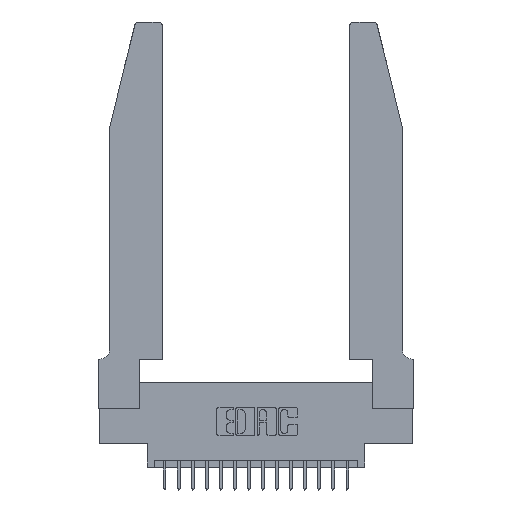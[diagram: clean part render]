
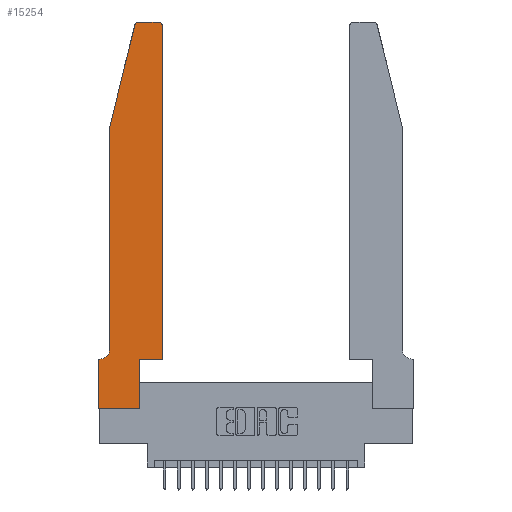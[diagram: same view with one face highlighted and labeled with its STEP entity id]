
A CAD part, top view. The second image highlights one B-rep face of the part: STEP entity #15254.
In plain terms, the highlighted planar face has unit normal (0, 0, 1).
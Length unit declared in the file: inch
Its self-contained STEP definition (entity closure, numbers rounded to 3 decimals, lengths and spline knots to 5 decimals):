
#12 = ORIENTED_EDGE ( 'NONE', *, *, #8720, .T. ) ;
#20 = CARTESIAN_POINT ( 'NONE',  ( 0.4505, 0.35, 0.37 ) ) ;
#29 = CARTESIAN_POINT ( 'NONE',  ( 0.0055, 0.35, 0.37 ) ) ;
#55 = CARTESIAN_POINT ( 'NONE',  ( 0., 0., 0.37 ) ) ;
#153 = LINE ( 'NONE', #2001, #19459 ) ;
#186 = VERTEX_POINT ( 'NONE', #4231 ) ;
#279 = ORIENTED_EDGE ( 'NONE', *, *, #2983, .T. ) ;
#730 = CARTESIAN_POINT ( 'NONE',  ( 0.2865, 0., 0.37 ) ) ;
#1021 = ORIENTED_EDGE ( 'NONE', *, *, #10683, .T. ) ;
#1034 = VERTEX_POINT ( 'NONE', #730 ) ;
#1045 = LINE ( 'NONE', #9131, #12900 ) ;
#1216 = VERTEX_POINT ( 'NONE', #13313 ) ;
#1297 = DIRECTION ( 'NONE',  ( 0., 1., 0. ) ) ;
#1299 = VECTOR ( 'NONE', #12445, 39.37008 ) ;
#1786 = ORIENTED_EDGE ( 'NONE', *, *, #2866, .T. ) ;
#1904 = ORIENTED_EDGE ( 'NONE', *, *, #4023, .T. ) ;
#2001 = CARTESIAN_POINT ( 'NONE',  ( 0., 0., 0.37 ) ) ;
#2242 = ORIENTED_EDGE ( 'NONE', *, *, #8294, .T. ) ;
#2747 = DIRECTION ( 'NONE',  ( -1., 0., 0. ) ) ;
#2837 = DIRECTION ( 'NONE',  ( 0., 0., 1. ) ) ;
#2853 = LINE ( 'NONE', #5395, #6052 ) ;
#2866 = EDGE_CURVE ( 'NONE', #18072, #1216, #2853, .T. ) ;
#2983 = EDGE_CURVE ( 'NONE', #17283, #18072, #4599, .T. ) ;
#3052 = VECTOR ( 'NONE', #2747, 39.37008 ) ;
#3189 = VECTOR ( 'NONE', #18941, 39.37008 ) ;
#3270 = VECTOR ( 'NONE', #19265, 39.37008 ) ;
#3274 = VERTEX_POINT ( 'NONE', #20 ) ;
#3355 = PLANE ( 'NONE',  #6150 ) ;
#3549 = LINE ( 'NONE', #4206, #3052 ) ;
#3795 = DIRECTION ( 'NONE',  ( 1., 0., 0. ) ) ;
#3819 = DIRECTION ( 'NONE',  ( 0., 0., 1. ) ) ;
#3846 = CARTESIAN_POINT ( 'NONE',  ( 0.284, 2.72, 0.37 ) ) ;
#4023 = EDGE_CURVE ( 'NONE', #4287, #186, #3549, .T. ) ;
#4206 = CARTESIAN_POINT ( 'NONE',  ( 0.0755, 0.35, 0.37 ) ) ;
#4231 = CARTESIAN_POINT ( 'NONE',  ( 0., 0.35, 0.37 ) ) ;
#4287 = VERTEX_POINT ( 'NONE', #29 ) ;
#4508 = VERTEX_POINT ( 'NONE', #18841 ) ;
#4599 = CIRCLE ( 'NONE', #12120, 0.03 ) ;
#4802 = CIRCLE ( 'NONE', #5574, 0.07 ) ;
#4921 = FACE_OUTER_BOUND ( 'NONE', #16742, .T. ) ;
#4939 = EDGE_CURVE ( 'NONE', #14732, #1034, #153, .T. ) ;
#4951 = DIRECTION ( 'NONE',  ( 0., 0., 1. ) ) ;
#5345 = DIRECTION ( 'NONE',  ( -0.239, -0.971, 0. ) ) ;
#5395 = CARTESIAN_POINT ( 'NONE',  ( 0.0755, 2., 0.37 ) ) ;
#5574 = AXIS2_PLACEMENT_3D ( 'NONE', #5576, #16064, #7082 ) ;
#5576 = CARTESIAN_POINT ( 'NONE',  ( 0.0055, 0.42, 0.37 ) ) ;
#5972 = AXIS2_PLACEMENT_3D ( 'NONE', #12069, #2837, #13557 ) ;
#6052 = VECTOR ( 'NONE', #5345, 39.37008 ) ;
#6150 = AXIS2_PLACEMENT_3D ( 'NONE', #14037, #4951, #15472 ) ;
#6274 = CARTESIAN_POINT ( 'NONE',  ( 0.4205, 2.75, 0.37 ) ) ;
#6568 = VECTOR ( 'NONE', #16923, 39.37008 ) ;
#7047 = CARTESIAN_POINT ( 'NONE',  ( 0.2865, 0.35, 0.37 ) ) ;
#7082 = DIRECTION ( 'NONE',  ( -1., 0., 0. ) ) ;
#7120 = CARTESIAN_POINT ( 'NONE',  ( 0.2605, 2.75, 0.37 ) ) ;
#7157 = ORIENTED_EDGE ( 'NONE', *, *, #9274, .T. ) ;
#7407 = LINE ( 'NONE', #7120, #3270 ) ;
#7699 = VERTEX_POINT ( 'NONE', #6274 ) ;
#8294 = EDGE_CURVE ( 'NONE', #4508, #3274, #1045, .T. ) ;
#8720 = EDGE_CURVE ( 'NONE', #12741, #4287, #4802, .T. ) ;
#9131 = CARTESIAN_POINT ( 'NONE',  ( 0.4505, 0.35, 0.37 ) ) ;
#9136 = LINE ( 'NONE', #19708, #1299 ) ;
#9274 = EDGE_CURVE ( 'NONE', #7699, #17283, #7407, .T. ) ;
#9313 = ORIENTED_EDGE ( 'NONE', *, *, #4939, .T. ) ;
#10466 = ORIENTED_EDGE ( 'NONE', *, *, #18468, .T. ) ;
#10553 = ORIENTED_EDGE ( 'NONE', *, *, #11905, .T. ) ;
#10683 = EDGE_CURVE ( 'NONE', #3274, #18572, #16045, .T. ) ;
#11286 = EDGE_CURVE ( 'NONE', #18572, #7699, #13765, .T. ) ;
#11905 = EDGE_CURVE ( 'NONE', #1034, #4508, #15308, .T. ) ;
#12069 = CARTESIAN_POINT ( 'NONE',  ( 0.4205, 2.72, 0.37 ) ) ;
#12120 = AXIS2_PLACEMENT_3D ( 'NONE', #3846, #3819, #3795 ) ;
#12445 = DIRECTION ( 'NONE',  ( 0., -1., 0. ) ) ;
#12741 = VERTEX_POINT ( 'NONE', #18030 ) ;
#12900 = VECTOR ( 'NONE', #19374, 39.37008 ) ;
#13313 = CARTESIAN_POINT ( 'NONE',  ( 0.0755, 2., 0.37 ) ) ;
#13379 = ORIENTED_EDGE ( 'NONE', *, *, #11286, .T. ) ;
#13557 = DIRECTION ( 'NONE',  ( 1., 0., 0. ) ) ;
#13605 = ORIENTED_EDGE ( 'NONE', *, *, #15824, .T. ) ;
#13765 = CIRCLE ( 'NONE', #5972, 0.03 ) ;
#14037 = CARTESIAN_POINT ( 'NONE',  ( 0., 0.35, 0.37 ) ) ;
#14732 = VERTEX_POINT ( 'NONE', #55 ) ;
#15254 = ADVANCED_FACE ( 'NONE', ( #4921 ), #3355, .T. ) ;
#15308 = LINE ( 'NONE', #7047, #3189 ) ;
#15357 = CARTESIAN_POINT ( 'NONE',  ( 0.284, 2.75, 0.37 ) ) ;
#15447 = CARTESIAN_POINT ( 'NONE',  ( 0., 0., 0.37 ) ) ;
#15472 = DIRECTION ( 'NONE',  ( 1., 0., 0. ) ) ;
#15556 = CARTESIAN_POINT ( 'NONE',  ( 0.4505, 2.72, 0.37 ) ) ;
#15824 = EDGE_CURVE ( 'NONE', #186, #14732, #18449, .T. ) ;
#15912 = CARTESIAN_POINT ( 'NONE',  ( 0.25487, 2.72718, 0.37 ) ) ;
#16045 = LINE ( 'NONE', #19406, #19454 ) ;
#16064 = DIRECTION ( 'NONE',  ( 0., 0., -1. ) ) ;
#16742 = EDGE_LOOP ( 'NONE', ( #7157, #279, #1786, #10466, #12, #1904, #13605, #9313, #10553, #2242, #1021, #13379 ) ) ;
#16923 = DIRECTION ( 'NONE',  ( 0., -1., 0. ) ) ;
#17283 = VERTEX_POINT ( 'NONE', #15357 ) ;
#18030 = CARTESIAN_POINT ( 'NONE',  ( 0.0755, 0.42, 0.37 ) ) ;
#18072 = VERTEX_POINT ( 'NONE', #15912 ) ;
#18449 = LINE ( 'NONE', #15447, #6568 ) ;
#18468 = EDGE_CURVE ( 'NONE', #1216, #12741, #9136, .T. ) ;
#18572 = VERTEX_POINT ( 'NONE', #15556 ) ;
#18633 = DIRECTION ( 'NONE',  ( 1., 0., 0. ) ) ;
#18841 = CARTESIAN_POINT ( 'NONE',  ( 0.2865, 0.35, 0.37 ) ) ;
#18941 = DIRECTION ( 'NONE',  ( 0., 1., 0. ) ) ;
#19265 = DIRECTION ( 'NONE',  ( -1., 0., 0. ) ) ;
#19374 = DIRECTION ( 'NONE',  ( 1., 0., 0. ) ) ;
#19406 = CARTESIAN_POINT ( 'NONE',  ( 0.4505, 0.35, 0.37 ) ) ;
#19454 = VECTOR ( 'NONE', #1297, 39.37008 ) ;
#19459 = VECTOR ( 'NONE', #18633, 39.37008 ) ;
#19708 = CARTESIAN_POINT ( 'NONE',  ( 0.0755, 2., 0.37 ) ) ;
